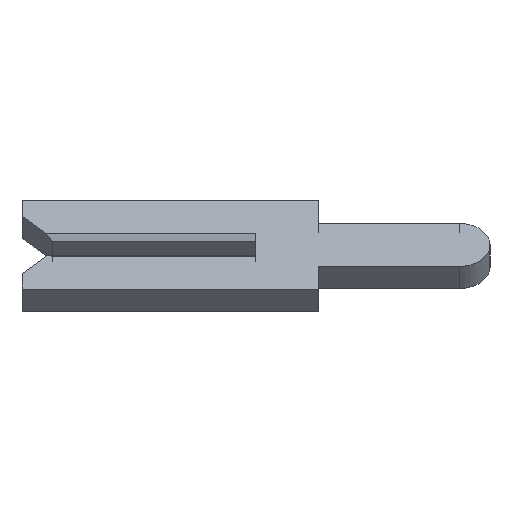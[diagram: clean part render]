
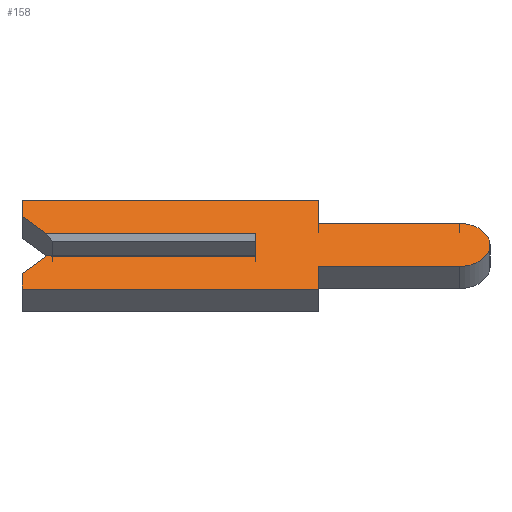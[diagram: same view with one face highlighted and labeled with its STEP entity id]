
A CAD part, left-side view. The second image highlights one B-rep face of the part: STEP entity #158.
In plain terms, the highlighted face is planar.
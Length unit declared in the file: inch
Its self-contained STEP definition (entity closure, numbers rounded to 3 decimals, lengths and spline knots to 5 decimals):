
#3 = DIRECTION ( 'NONE',  ( 0., 0., -1. ) ) ;
#15 = CARTESIAN_POINT ( 'NONE',  ( -0.01, -0.04, -0.04 ) ) ;
#18 = EDGE_CURVE ( 'NONE', #76, #996, #796, .T. ) ;
#29 = CARTESIAN_POINT ( 'NONE',  ( -0.01, -0.04, 0.04 ) ) ;
#40 = VERTEX_POINT ( 'NONE', #913 ) ;
#41 = CARTESIAN_POINT ( 'NONE',  ( -0.01, 0., 0.0065 ) ) ;
#47 = DIRECTION ( 'NONE',  ( 0., 0., 1. ) ) ;
#51 = VECTOR ( 'NONE', #758, 39.37008 ) ;
#60 = EDGE_CURVE ( 'NONE', #1141, #40, #1262, .T. ) ;
#70 = DIRECTION ( 'NONE',  ( 0., 1., 0. ) ) ;
#76 = VERTEX_POINT ( 'NONE', #612 ) ;
#120 = VECTOR ( 'NONE', #638, 39.37008 ) ;
#123 = LINE ( 'NONE', #124, #563 ) ;
#124 = CARTESIAN_POINT ( 'NONE',  ( -0.01, 0.15, 0.01 ) ) ;
#139 = VECTOR ( 'NONE', #47, 39.37008 ) ;
#155 = CARTESIAN_POINT ( 'NONE',  ( -0.01, 0.15, 0.026 ) ) ;
#158 = ADVANCED_FACE ( 'NONE', ( #526 ), #393, .F. ) ;
#179 = AXIS2_PLACEMENT_3D ( 'NONE', #867, #872, #549 ) ;
#199 = VERTEX_POINT ( 'NONE', #15 ) ;
#206 = DIRECTION ( 'NONE',  ( 1., 0., 0. ) ) ;
#218 = LINE ( 'NONE', #803, #1063 ) ;
#233 = ORIENTED_EDGE ( 'NONE', *, *, #530, .F. ) ;
#264 = VERTEX_POINT ( 'NONE', #945 ) ;
#308 = EDGE_CURVE ( 'NONE', #1078, #587, #574, .T. ) ;
#319 = CARTESIAN_POINT ( 'NONE',  ( -0.01, 0.1305, -0.0065 ) ) ;
#324 = CARTESIAN_POINT ( 'NONE',  ( -0.01, 0.134, -0.01 ) ) ;
#334 = DIRECTION ( 'NONE',  ( 0., 0., 1. ) ) ;
#354 = CARTESIAN_POINT ( 'NONE',  ( -0.01, 0.15, -0.04 ) ) ;
#366 = CARTESIAN_POINT ( 'NONE',  ( -0.01, -0.1305, -0.0195 ) ) ;
#372 = VERTEX_POINT ( 'NONE', #628 ) ;
#376 = ORIENTED_EDGE ( 'NONE', *, *, #308, .F. ) ;
#390 = DIRECTION ( 'NONE',  ( 0., -1., 0. ) ) ;
#393 = PLANE ( 'NONE',  #615 ) ;
#421 = ORIENTED_EDGE ( 'NONE', *, *, #1246, .F. ) ;
#422 = ORIENTED_EDGE ( 'NONE', *, *, #522, .F. ) ;
#426 = DIRECTION ( 'NONE',  ( 0., 0., -1. ) ) ;
#447 = EDGE_CURVE ( 'NONE', #40, #613, #510, .T. ) ;
#458 = LINE ( 'NONE', #1122, #1218 ) ;
#459 = VECTOR ( 'NONE', #334, 39.37008 ) ;
#472 = EDGE_LOOP ( 'NONE', ( #1104, #233, #963, #376, #422, #997, #1061, #584, #896, #421, #573, #912, #958, #732 ) ) ;
#473 = EDGE_CURVE ( 'NONE', #76, #372, #123, .T. ) ;
#477 = EDGE_CURVE ( 'NONE', #264, #779, #798, .T. ) ;
#502 = DIRECTION ( 'NONE',  ( 0., 0., -1. ) ) ;
#510 = LINE ( 'NONE', #29, #623 ) ;
#517 = CARTESIAN_POINT ( 'NONE',  ( -0.01, 0.1305, 0.0065 ) ) ;
#522 = EDGE_CURVE ( 'NONE', #775, #1078, #966, .T. ) ;
#526 = FACE_OUTER_BOUND ( 'NONE', #472, .T. ) ;
#530 = EDGE_CURVE ( 'NONE', #618, #372, #886, .T. ) ;
#536 = LINE ( 'NONE', #578, #1286 ) ;
#546 = VERTEX_POINT ( 'NONE', #1278 ) ;
#549 = DIRECTION ( 'NONE',  ( 0., 0., -1. ) ) ;
#553 = CARTESIAN_POINT ( 'NONE',  ( -0.01, 0., -0.01 ) ) ;
#563 = VECTOR ( 'NONE', #851, 39.37008 ) ;
#573 = ORIENTED_EDGE ( 'NONE', *, *, #447, .F. ) ;
#574 = LINE ( 'NONE', #319, #120 ) ;
#578 = CARTESIAN_POINT ( 'NONE',  ( -0.01, -0.04, -0.0195 ) ) ;
#584 = ORIENTED_EDGE ( 'NONE', *, *, #968, .F. ) ;
#587 = VERTEX_POINT ( 'NONE', #324 ) ;
#612 = CARTESIAN_POINT ( 'NONE',  ( -0.01, 0.134, 0.01 ) ) ;
#613 = VERTEX_POINT ( 'NONE', #860 ) ;
#615 = AXIS2_PLACEMENT_3D ( 'NONE', #706, #206, #502 ) ;
#618 = VERTEX_POINT ( 'NONE', #553 ) ;
#623 = VECTOR ( 'NONE', #426, 39.37008 ) ;
#628 = CARTESIAN_POINT ( 'NONE',  ( -0.01, 0., 0.01 ) ) ;
#629 = EDGE_CURVE ( 'NONE', #199, #775, #1149, .T. ) ;
#638 = DIRECTION ( 'NONE',  ( 0., -0.707, 0.707 ) ) ;
#658 = CARTESIAN_POINT ( 'NONE',  ( -0.01, 0.15, -0.026 ) ) ;
#670 = DIRECTION ( 'NONE',  ( 0., 0., 1. ) ) ;
#704 = DIRECTION ( 'NONE',  ( 0., 0.707, 0.707 ) ) ;
#706 = CARTESIAN_POINT ( 'NONE',  ( -0.01, -0.1305, 0. ) ) ;
#732 = ORIENTED_EDGE ( 'NONE', *, *, #18, .F. ) ;
#736 = LINE ( 'NONE', #1205, #841 ) ;
#758 = DIRECTION ( 'NONE',  ( 0., 1., 0. ) ) ;
#772 = EDGE_CURVE ( 'NONE', #996, #1141, #817, .T. ) ;
#775 = VERTEX_POINT ( 'NONE', #354 ) ;
#777 = DIRECTION ( 'NONE',  ( 0., -1., 0. ) ) ;
#779 = VERTEX_POINT ( 'NONE', #366 ) ;
#780 = VECTOR ( 'NONE', #670, 39.37008 ) ;
#796 = LINE ( 'NONE', #517, #1238 ) ;
#798 = CIRCLE ( 'NONE', #179, 0.0195 ) ;
#803 = CARTESIAN_POINT ( 'NONE',  ( -0.01, -0.04, -0.04 ) ) ;
#817 = LINE ( 'NONE', #1198, #780 ) ;
#841 = VECTOR ( 'NONE', #777, 39.37008 ) ;
#851 = DIRECTION ( 'NONE',  ( 0., -1., 0. ) ) ;
#860 = CARTESIAN_POINT ( 'NONE',  ( -0.01, -0.04, 0.0195 ) ) ;
#867 = CARTESIAN_POINT ( 'NONE',  ( -0.01, -0.1305, 0. ) ) ;
#872 = DIRECTION ( 'NONE',  ( 1., 0., 0. ) ) ;
#886 = LINE ( 'NONE', #41, #139 ) ;
#896 = ORIENTED_EDGE ( 'NONE', *, *, #477, .F. ) ;
#900 = CARTESIAN_POINT ( 'NONE',  ( -0.01, 0.15, 0.04 ) ) ;
#912 = ORIENTED_EDGE ( 'NONE', *, *, #60, .F. ) ;
#913 = CARTESIAN_POINT ( 'NONE',  ( -0.01, -0.04, 0.04 ) ) ;
#919 = DIRECTION ( 'NONE',  ( 0., -1., 0. ) ) ;
#939 = EDGE_CURVE ( 'NONE', #587, #618, #736, .T. ) ;
#945 = CARTESIAN_POINT ( 'NONE',  ( -0.01, -0.1305, 0.0195 ) ) ;
#958 = ORIENTED_EDGE ( 'NONE', *, *, #772, .F. ) ;
#963 = ORIENTED_EDGE ( 'NONE', *, *, #939, .F. ) ;
#966 = LINE ( 'NONE', #658, #459 ) ;
#968 = EDGE_CURVE ( 'NONE', #779, #546, #536, .T. ) ;
#981 = VECTOR ( 'NONE', #919, 39.37008 ) ;
#996 = VERTEX_POINT ( 'NONE', #155 ) ;
#997 = ORIENTED_EDGE ( 'NONE', *, *, #629, .F. ) ;
#1016 = CARTESIAN_POINT ( 'NONE',  ( -0.01, 0.15, 0.04 ) ) ;
#1061 = ORIENTED_EDGE ( 'NONE', *, *, #1191, .F. ) ;
#1063 = VECTOR ( 'NONE', #3, 39.37008 ) ;
#1068 = CARTESIAN_POINT ( 'NONE',  ( -0.01, 0.15, -0.04 ) ) ;
#1078 = VERTEX_POINT ( 'NONE', #1107 ) ;
#1104 = ORIENTED_EDGE ( 'NONE', *, *, #473, .T. ) ;
#1107 = CARTESIAN_POINT ( 'NONE',  ( -0.01, 0.15, -0.026 ) ) ;
#1122 = CARTESIAN_POINT ( 'NONE',  ( -0.01, -0.04, 0.0195 ) ) ;
#1141 = VERTEX_POINT ( 'NONE', #900 ) ;
#1149 = LINE ( 'NONE', #1068, #51 ) ;
#1191 = EDGE_CURVE ( 'NONE', #546, #199, #218, .T. ) ;
#1198 = CARTESIAN_POINT ( 'NONE',  ( -0.01, 0.15, 0.026 ) ) ;
#1205 = CARTESIAN_POINT ( 'NONE',  ( -0.01, -0.1305, -0.01 ) ) ;
#1218 = VECTOR ( 'NONE', #390, 39.37008 ) ;
#1238 = VECTOR ( 'NONE', #704, 39.37008 ) ;
#1246 = EDGE_CURVE ( 'NONE', #613, #264, #458, .T. ) ;
#1262 = LINE ( 'NONE', #1016, #981 ) ;
#1278 = CARTESIAN_POINT ( 'NONE',  ( -0.01, -0.04, -0.0195 ) ) ;
#1286 = VECTOR ( 'NONE', #70, 39.37008 ) ;
